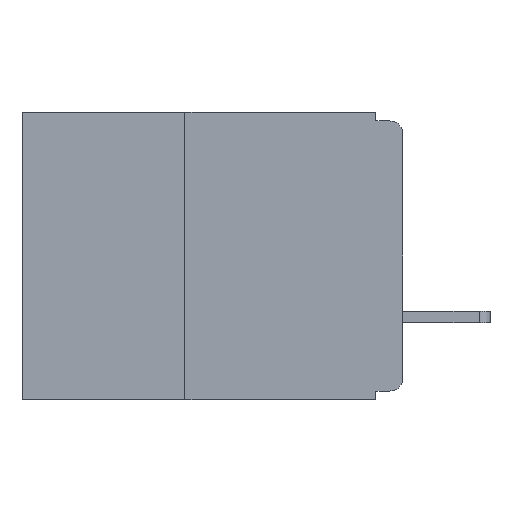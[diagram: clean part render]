
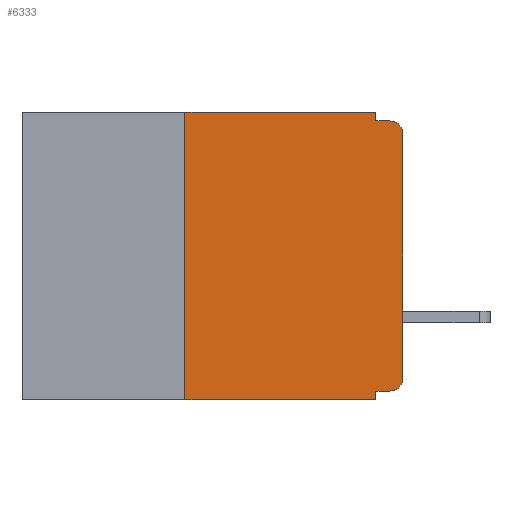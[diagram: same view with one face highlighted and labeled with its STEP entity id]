
A CAD part, left-side view. The second image highlights one B-rep face of the part: STEP entity #6333.
In plain terms, the highlighted planar face has unit normal (-1, 0, 0).
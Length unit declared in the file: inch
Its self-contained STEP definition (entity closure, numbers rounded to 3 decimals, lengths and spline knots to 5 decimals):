
#337 = VERTEX_POINT ( 'NONE', #20287 ) ;
#580 = ORIENTED_EDGE ( 'NONE', *, *, #11748, .T. ) ;
#1377 = DIRECTION ( 'NONE',  ( 0., 0., -1. ) ) ;
#1592 = VERTEX_POINT ( 'NONE', #5553 ) ;
#1873 = EDGE_CURVE ( 'NONE', #11133, #3860, #4439, .T. ) ;
#2184 = VERTEX_POINT ( 'NONE', #15270 ) ;
#2667 = CARTESIAN_POINT ( 'NONE',  ( 0., 0.015, -0.305 ) ) ;
#3251 = DIRECTION ( 'NONE',  ( 0., 0., 1. ) ) ;
#3261 = DIRECTION ( 'NONE',  ( 0., 1., 0. ) ) ;
#3323 = EDGE_CURVE ( 'NONE', #24658, #3870, #14860, .T. ) ;
#3860 = VERTEX_POINT ( 'NONE', #24835 ) ;
#3870 = VERTEX_POINT ( 'NONE', #24075 ) ;
#3972 = LINE ( 'NONE', #8634, #24267 ) ;
#4013 = EDGE_CURVE ( 'NONE', #337, #2184, #10217, .T. ) ;
#4114 = ORIENTED_EDGE ( 'NONE', *, *, #14329, .F. ) ;
#4439 = LINE ( 'NONE', #22842, #9155 ) ;
#4649 = DIRECTION ( 'NONE',  ( 0., 0., -1. ) ) ;
#4667 = DIRECTION ( 'NONE',  ( 0., 0., -1. ) ) ;
#5295 = CARTESIAN_POINT ( 'NONE',  ( 0., 0.031, -0.33 ) ) ;
#5426 = CARTESIAN_POINT ( 'NONE',  ( 0., 0.015, -0.32 ) ) ;
#5483 = VECTOR ( 'NONE', #14495, 39.37008 ) ;
#5553 = CARTESIAN_POINT ( 'NONE',  ( 0., 0.031, -0.32 ) ) ;
#6333 = ADVANCED_FACE ( 'NONE', ( #6911 ), #7292, .F. ) ;
#6849 = ORIENTED_EDGE ( 'NONE', *, *, #24703, .T. ) ;
#6911 = FACE_OUTER_BOUND ( 'NONE', #8128, .T. ) ;
#7245 = DIRECTION ( 'NONE',  ( -1., 0., 0. ) ) ;
#7292 = PLANE ( 'NONE',  #9379 ) ;
#7320 = DIRECTION ( 'NONE',  ( 0., 0., -1. ) ) ;
#7445 = LINE ( 'NONE', #15085, #12144 ) ;
#7523 = CARTESIAN_POINT ( 'NONE',  ( 0., 0.25, -0.33 ) ) ;
#7702 = ORIENTED_EDGE ( 'NONE', *, *, #10032, .F. ) ;
#8128 = EDGE_LOOP ( 'NONE', ( #20916, #580, #8400, #4114, #24020, #15848, #6849, #7702, #18662, #19195 ) ) ;
#8400 = ORIENTED_EDGE ( 'NONE', *, *, #3323, .F. ) ;
#8456 = AXIS2_PLACEMENT_3D ( 'NONE', #18949, #7245, #20924 ) ;
#8634 = CARTESIAN_POINT ( 'NONE',  ( 0., 0.031, 0. ) ) ;
#8781 = EDGE_CURVE ( 'NONE', #17349, #337, #7445, .T. ) ;
#9155 = VECTOR ( 'NONE', #22171, 39.37008 ) ;
#9379 = AXIS2_PLACEMENT_3D ( 'NONE', #18992, #13269, #1377 ) ;
#9802 = VECTOR ( 'NONE', #3261, 39.37008 ) ;
#10032 = EDGE_CURVE ( 'NONE', #1592, #11437, #12301, .T. ) ;
#10121 = CIRCLE ( 'NONE', #23227, 0.015 ) ;
#10217 = LINE ( 'NONE', #14786, #5483 ) ;
#10317 = LINE ( 'NONE', #23280, #25274 ) ;
#11133 = VERTEX_POINT ( 'NONE', #22510 ) ;
#11437 = VERTEX_POINT ( 'NONE', #19887 ) ;
#11709 = VECTOR ( 'NONE', #7320, 39.37008 ) ;
#11748 = EDGE_CURVE ( 'NONE', #3860, #3870, #12204, .T. ) ;
#11804 = CARTESIAN_POINT ( 'NONE',  ( 0., 0., -0.01 ) ) ;
#12144 = VECTOR ( 'NONE', #3251, 39.37008 ) ;
#12204 = CIRCLE ( 'NONE', #8456, 0.015 ) ;
#12301 = LINE ( 'NONE', #5295, #11709 ) ;
#13269 = DIRECTION ( 'NONE',  ( 1., 0., 0. ) ) ;
#13578 = DIRECTION ( 'NONE',  ( 0., -1., 0. ) ) ;
#14329 = EDGE_CURVE ( 'NONE', #2184, #24658, #3972, .T. ) ;
#14495 = DIRECTION ( 'NONE',  ( 0., -1., 0. ) ) ;
#14786 = CARTESIAN_POINT ( 'NONE',  ( 0., 0.437, 0. ) ) ;
#14860 = LINE ( 'NONE', #11804, #22802 ) ;
#15085 = CARTESIAN_POINT ( 'NONE',  ( 0., 0.25, -0.33 ) ) ;
#15270 = CARTESIAN_POINT ( 'NONE',  ( 0., 0.031, 0. ) ) ;
#15848 = ORIENTED_EDGE ( 'NONE', *, *, #8781, .F. ) ;
#16450 = DIRECTION ( 'NONE',  ( -1., 0., 0. ) ) ;
#17039 = CARTESIAN_POINT ( 'NONE',  ( 0., 0., -0.32 ) ) ;
#17349 = VERTEX_POINT ( 'NONE', #7523 ) ;
#18662 = ORIENTED_EDGE ( 'NONE', *, *, #23028, .F. ) ;
#18949 = CARTESIAN_POINT ( 'NONE',  ( 0., 0.015, -0.025 ) ) ;
#18992 = CARTESIAN_POINT ( 'NONE',  ( 0., 0.437, 0. ) ) ;
#19195 = ORIENTED_EDGE ( 'NONE', *, *, #22847, .T. ) ;
#19858 = DIRECTION ( 'NONE',  ( 0., -1., 0. ) ) ;
#19887 = CARTESIAN_POINT ( 'NONE',  ( 0., 0.031, -0.33 ) ) ;
#20287 = CARTESIAN_POINT ( 'NONE',  ( 0., 0.25, 0. ) ) ;
#20916 = ORIENTED_EDGE ( 'NONE', *, *, #1873, .T. ) ;
#20924 = DIRECTION ( 'NONE',  ( 0., 0., -1. ) ) ;
#22171 = DIRECTION ( 'NONE',  ( 0., 0., 1. ) ) ;
#22510 = CARTESIAN_POINT ( 'NONE',  ( 0., 0., -0.305 ) ) ;
#22802 = VECTOR ( 'NONE', #19858, 39.37008 ) ;
#22842 = CARTESIAN_POINT ( 'NONE',  ( 0., 0., 0. ) ) ;
#22847 = EDGE_CURVE ( 'NONE', #23097, #11133, #10121, .T. ) ;
#23028 = EDGE_CURVE ( 'NONE', #23097, #1592, #24751, .T. ) ;
#23097 = VERTEX_POINT ( 'NONE', #5426 ) ;
#23197 = CARTESIAN_POINT ( 'NONE',  ( 0., 0.031, -0.01 ) ) ;
#23227 = AXIS2_PLACEMENT_3D ( 'NONE', #2667, #16450, #4649 ) ;
#23280 = CARTESIAN_POINT ( 'NONE',  ( 0., 0.437, -0.33 ) ) ;
#24020 = ORIENTED_EDGE ( 'NONE', *, *, #4013, .F. ) ;
#24075 = CARTESIAN_POINT ( 'NONE',  ( 0., 0.015, -0.01 ) ) ;
#24267 = VECTOR ( 'NONE', #4667, 39.37008 ) ;
#24658 = VERTEX_POINT ( 'NONE', #23197 ) ;
#24703 = EDGE_CURVE ( 'NONE', #17349, #11437, #10317, .T. ) ;
#24751 = LINE ( 'NONE', #17039, #9802 ) ;
#24835 = CARTESIAN_POINT ( 'NONE',  ( 0., 0., -0.025 ) ) ;
#25274 = VECTOR ( 'NONE', #13578, 39.37008 ) ;
